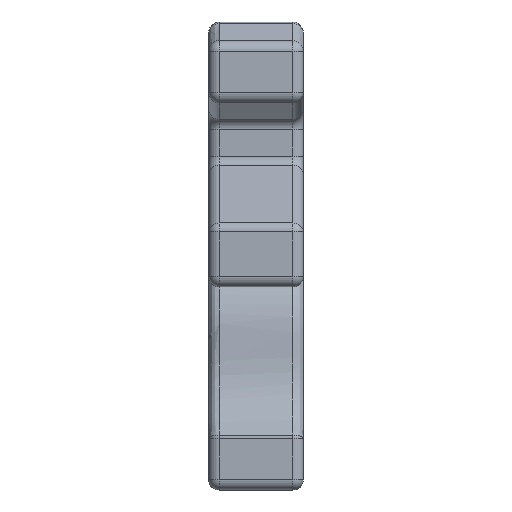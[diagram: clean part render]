
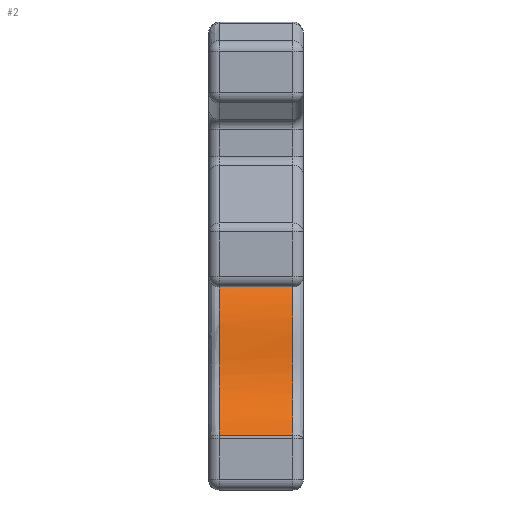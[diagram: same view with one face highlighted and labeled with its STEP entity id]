
A CAD part, front view. The second image highlights one B-rep face of the part: STEP entity #2.
In plain terms, the highlighted free-form (B-spline) face has degree [3, 1] with [4, 2] control points.
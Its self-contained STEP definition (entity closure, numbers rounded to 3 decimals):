
#2 = ADVANCED_FACE ( 'NONE', ( #2092 ), #1646, .T. ) ;
#130 = EDGE_CURVE ( 'NONE', #1262, #1258, #2833, .T. ) ;
#132 = EDGE_CURVE ( 'NONE', #1267, #1271, #2842, .T. ) ;
#134 = EDGE_CURVE ( 'NONE', #1271, #1262, #2474, .T. ) ;
#136 = EDGE_CURVE ( 'NONE', #1258, #1267, #2479, .T. ) ;
#767 = ORIENTED_EDGE ( 'NONE', *, *, #134, .T. ) ;
#776 = ORIENTED_EDGE ( 'NONE', *, *, #136, .T. ) ;
#787 = ORIENTED_EDGE ( 'NONE', *, *, #130, .T. ) ;
#806 = ORIENTED_EDGE ( 'NONE', *, *, #132, .T. ) ;
#1258 = VERTEX_POINT ( 'NONE', #2215 ) ;
#1262 = VERTEX_POINT ( 'NONE', #2218 ) ;
#1267 = VERTEX_POINT ( 'NONE', #2221 ) ;
#1271 = VERTEX_POINT ( 'NONE', #2224 ) ;
#1646 = B_SPLINE_SURFACE_WITH_KNOTS ( 'NONE', 3, 1, ( 
 ( #3653, #3672 ),
 ( #3657, #3663 ),
 ( #3675, #3666 ),
 ( #3668, #3674 ) ),
 .UNSPECIFIED., .F., .F., .F.,
 ( 4, 4 ),
 ( 2, 2 ),
 ( 0.005, 0.97 ),
 ( 0., 1. ),
 .UNSPECIFIED. ) ;
#2020 = EDGE_LOOP ( 'NONE', ( #806, #767, #787, #776 ) ) ;
#2092 = FACE_OUTER_BOUND ( 'NONE', #2020, .T. ) ;
#2215 = CARTESIAN_POINT ( 'NONE',  ( 1., 12.514, -11.656 ) ) ;
#2218 = CARTESIAN_POINT ( 'NONE',  ( 8., 12.514, -11.656 ) ) ;
#2221 = CARTESIAN_POINT ( 'NONE',  ( 1., -9.591, -30.658 ) ) ;
#2224 = CARTESIAN_POINT ( 'NONE',  ( 8., -9.591, -30.658 ) ) ;
#2474 = B_SPLINE_CURVE_WITH_KNOTS ( 'NONE', 3,
 ( #3046, #3041, #3040, #3047, #3048, #3049, #3050, #3051, #3052, #3053, #3054, #3055, #3056, #3057, #3058, #3059, #3060, #3061, #3062, #3063, #3064, #3065, #3066, #3067, #3068, #3069, #3070, #3071, #3072, #3073, #3074, #3075, #3076, #3077 ),
 .UNSPECIFIED., .F., .F.,
 ( 4, 2, 2, 2, 2, 2, 2, 2, 2, 2, 2, 2, 2, 2, 2, 2, 4 ),
 ( 0., 0.002, 0.003, 0.004, 0.006, 0.008, 0.011, 0.015, 0.017, 0.019, 0.023, 0.024, 0.025, 0.027, 0.028, 0.029, 0.031 ),
 .UNSPECIFIED. ) ;
#2479 = B_SPLINE_CURVE_WITH_KNOTS ( 'NONE', 3,
 ( #3080, #3042, #3035, #3081, #3082, #3083, #3084, #3085, #3086, #3087, #3088, #3089, #3090, #3091, #3092, #3093, #3094, #3095, #3096, #3097, #3098, #3099, #3100, #3101, #3102, #3103, #3104, #3105, #3106, #3107 ),
 .UNSPECIFIED., .F., .F.,
 ( 4, 2, 2, 2, 2, 2, 2, 2, 2, 2, 2, 2, 2, 2, 4 ),
 ( 0., 0.002, 0.003, 0.004, 0.006, 0.007, 0.008, 0.012, 0.015, 0.019, 0.023, 0.027, 0.029, 0.03, 0.031 ),
 .UNSPECIFIED. ) ;
#2704 = VECTOR ( 'NONE', #3034, 1000. ) ;
#2833 = LINE ( 'NONE', #3030, #2841 ) ;
#2841 = VECTOR ( 'NONE', #3033, 1000. ) ;
#2842 = LINE ( 'NONE', #3036, #2704 ) ;
#3030 = CARTESIAN_POINT ( 'NONE',  ( 9., 12.514, -11.656 ) ) ;
#3033 = DIRECTION ( 'NONE',  ( -1., 0., 0. ) ) ;
#3034 = DIRECTION ( 'NONE',  ( 1., 0., 0. ) ) ;
#3035 = CARTESIAN_POINT ( 'NONE',  ( 1., 12.29, -12.924 ) ) ;
#3036 = CARTESIAN_POINT ( 'NONE',  ( 0., -9.591, -30.658 ) ) ;
#3040 = CARTESIAN_POINT ( 'NONE',  ( 8., -9.101, -29.478 ) ) ;
#3041 = CARTESIAN_POINT ( 'NONE',  ( 8., -9.374, -30.055 ) ) ;
#3042 = CARTESIAN_POINT ( 'NONE',  ( 1., 12.426, -12.297 ) ) ;
#3046 = CARTESIAN_POINT ( 'NONE',  ( 8., -9.591, -30.658 ) ) ;
#3047 = CARTESIAN_POINT ( 'NONE',  ( 8., -8.607, -28.657 ) ) ;
#3048 = CARTESIAN_POINT ( 'NONE',  ( 8., -8.427, -28.39 ) ) ;
#3049 = CARTESIAN_POINT ( 'NONE',  ( 8., -8.048, -27.881 ) ) ;
#3050 = CARTESIAN_POINT ( 'NONE',  ( 8., -7.847, -27.637 ) ) ;
#3051 = CARTESIAN_POINT ( 'NONE',  ( 8., -7.212, -26.933 ) ) ;
#3052 = CARTESIAN_POINT ( 'NONE',  ( 8., -6.747, -26.502 ) ) ;
#3053 = CARTESIAN_POINT ( 'NONE',  ( 8., -5.748, -25.704 ) ) ;
#3054 = CARTESIAN_POINT ( 'NONE',  ( 8., -5.225, -25.344 ) ) ;
#3055 = CARTESIAN_POINT ( 'NONE',  ( 8., -3.604, -24.347 ) ) ;
#3056 = CARTESIAN_POINT ( 'NONE',  ( 8., -2.455, -23.79 ) ) ;
#3057 = CARTESIAN_POINT ( 'NONE',  ( 8., -0.126, -22.762 ) ) ;
#3058 = CARTESIAN_POINT ( 'NONE',  ( 8., 1.058, -22.291 ) ) ;
#3059 = CARTESIAN_POINT ( 'NONE',  ( 8., 2.823, -21.56 ) ) ;
#3060 = CARTESIAN_POINT ( 'NONE',  ( 8., 3.409, -21.312 ) ) ;
#3061 = CARTESIAN_POINT ( 'NONE',  ( 8., 4.572, -20.793 ) ) ;
#3062 = CARTESIAN_POINT ( 'NONE',  ( 8., 5.149, -20.521 ) ) ;
#3063 = CARTESIAN_POINT ( 'NONE',  ( 8., 6.847, -19.647 ) ) ;
#3064 = CARTESIAN_POINT ( 'NONE',  ( 8., 7.929, -18.99 ) ) ;
#3065 = CARTESIAN_POINT ( 'NONE',  ( 8., 9.151, -17.972 ) ) ;
#3066 = CARTESIAN_POINT ( 'NONE',  ( 8., 9.389, -17.758 ) ) ;
#3067 = CARTESIAN_POINT ( 'NONE',  ( 8., 9.846, -17.309 ) ) ;
#3068 = CARTESIAN_POINT ( 'NONE',  ( 8., 10.063, -17.076 ) ) ;
#3069 = CARTESIAN_POINT ( 'NONE',  ( 8., 10.678, -16.351 ) ) ;
#3070 = CARTESIAN_POINT ( 'NONE',  ( 8., 11.04, -15.832 ) ) ;
#3071 = CARTESIAN_POINT ( 'NONE',  ( 8., 11.504, -14.993 ) ) ;
#3072 = CARTESIAN_POINT ( 'NONE',  ( 8., 11.645, -14.703 ) ) ;
#3073 = CARTESIAN_POINT ( 'NONE',  ( 8., 11.895, -14.117 ) ) ;
#3074 = CARTESIAN_POINT ( 'NONE',  ( 8., 12.005, -13.819 ) ) ;
#3075 = CARTESIAN_POINT ( 'NONE',  ( 8., 12.292, -12.913 ) ) ;
#3076 = CARTESIAN_POINT ( 'NONE',  ( 8., 12.427, -12.292 ) ) ;
#3077 = CARTESIAN_POINT ( 'NONE',  ( 8., 12.514, -11.656 ) ) ;
#3080 = CARTESIAN_POINT ( 'NONE',  ( 1., 12.514, -11.656 ) ) ;
#3081 = CARTESIAN_POINT ( 'NONE',  ( 1., 11.998, -13.839 ) ) ;
#3082 = CARTESIAN_POINT ( 'NONE',  ( 1., 11.887, -14.14 ) ) ;
#3083 = CARTESIAN_POINT ( 'NONE',  ( 1., 11.632, -14.732 ) ) ;
#3084 = CARTESIAN_POINT ( 'NONE',  ( 1., 11.488, -15.024 ) ) ;
#3085 = CARTESIAN_POINT ( 'NONE',  ( 1., 11.019, -15.865 ) ) ;
#3086 = CARTESIAN_POINT ( 'NONE',  ( 1., 10.652, -16.387 ) ) ;
#3087 = CARTESIAN_POINT ( 'NONE',  ( 1., 10.026, -17.117 ) ) ;
#3088 = CARTESIAN_POINT ( 'NONE',  ( 1., 9.805, -17.351 ) ) ;
#3089 = CARTESIAN_POINT ( 'NONE',  ( 1., 9.341, -17.802 ) ) ;
#3090 = CARTESIAN_POINT ( 'NONE',  ( 1., 9.102, -18.014 ) ) ;
#3091 = CARTESIAN_POINT ( 'NONE',  ( 1., 7.876, -19.026 ) ) ;
#3092 = CARTESIAN_POINT ( 'NONE',  ( 1., 6.798, -19.674 ) ) ;
#3093 = CARTESIAN_POINT ( 'NONE',  ( 1., 4.557, -20.824 ) ) ;
#3094 = CARTESIAN_POINT ( 'NONE',  ( 1., 3.391, -21.324 ) ) ;
#3095 = CARTESIAN_POINT ( 'NONE',  ( 1., 1.046, -22.296 ) ) ;
#3096 = CARTESIAN_POINT ( 'NONE',  ( 1., -0.134, -22.765 ) ) ;
#3097 = CARTESIAN_POINT ( 'NONE',  ( 1., -2.455, -23.79 ) ) ;
#3098 = CARTESIAN_POINT ( 'NONE',  ( 1., -3.597, -24.342 ) ) ;
#3099 = CARTESIAN_POINT ( 'NONE',  ( 1., -5.772, -25.681 ) ) ;
#3100 = CARTESIAN_POINT ( 'NONE',  ( 1., -6.781, -26.454 ) ) ;
#3101 = CARTESIAN_POINT ( 'NONE',  ( 1., -8.068, -27.883 ) ) ;
#3102 = CARTESIAN_POINT ( 'NONE',  ( 1., -8.446, -28.391 ) ) ;
#3103 = CARTESIAN_POINT ( 'NONE',  ( 1., -8.936, -29.203 ) ) ;
#3104 = CARTESIAN_POINT ( 'NONE',  ( 1., -9.086, -29.483 ) ) ;
#3105 = CARTESIAN_POINT ( 'NONE',  ( 1., -9.359, -30.059 ) ) ;
#3106 = CARTESIAN_POINT ( 'NONE',  ( 1., -9.482, -30.356 ) ) ;
#3107 = CARTESIAN_POINT ( 'NONE',  ( 1., -9.591, -30.658 ) ) ;
#3653 = CARTESIAN_POINT ( 'NONE',  ( 8., -9.591, -30.658 ) ) ;
#3657 = CARTESIAN_POINT ( 'NONE',  ( 8., -5.963, -20.597 ) ) ;
#3663 = CARTESIAN_POINT ( 'NONE',  ( 1., -5.963, -20.597 ) ) ;
#3666 = CARTESIAN_POINT ( 'NONE',  ( 1., 10.898, -23.461 ) ) ;
#3668 = CARTESIAN_POINT ( 'NONE',  ( 8., 12.514, -11.656 ) ) ;
#3672 = CARTESIAN_POINT ( 'NONE',  ( 1., -9.591, -30.658 ) ) ;
#3674 = CARTESIAN_POINT ( 'NONE',  ( 1., 12.514, -11.656 ) ) ;
#3675 = CARTESIAN_POINT ( 'NONE',  ( 8., 10.898, -23.461 ) ) ;
